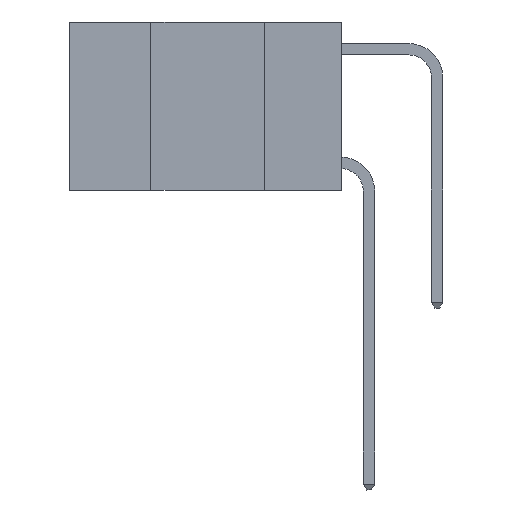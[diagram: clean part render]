
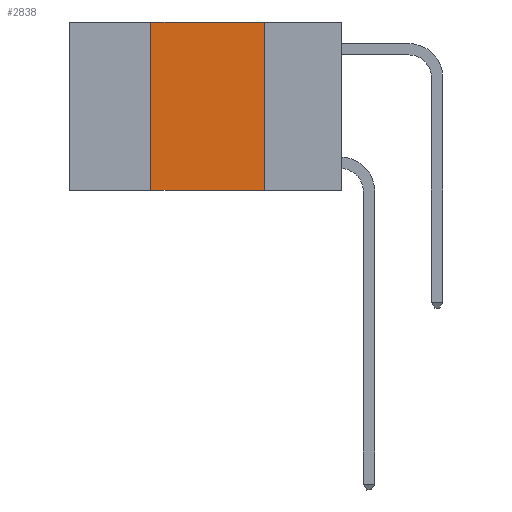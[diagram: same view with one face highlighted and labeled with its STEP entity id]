
A CAD part, left-side view. The second image highlights one B-rep face of the part: STEP entity #2838.
In plain terms, the highlighted planar face has unit normal (-1, 0, 0).
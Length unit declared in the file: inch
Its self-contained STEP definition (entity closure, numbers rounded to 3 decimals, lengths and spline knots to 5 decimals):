
#393 = ORIENTED_EDGE ( 'NONE', *, *, #5896, .T. ) ;
#488 = VECTOR ( 'NONE', #11112, 39.37008 ) ;
#521 = CARTESIAN_POINT ( 'NONE',  ( 0., 0.17, 0. ) ) ;
#688 = ORIENTED_EDGE ( 'NONE', *, *, #948, .F. ) ;
#948 = EDGE_CURVE ( 'NONE', #10338, #5953, #5737, .T. ) ;
#1425 = EDGE_LOOP ( 'NONE', ( #688, #5226, #4576, #393 ) ) ;
#1478 = EDGE_CURVE ( 'NONE', #5827, #5379, #10811, .T. ) ;
#2143 = LINE ( 'NONE', #10212, #6432 ) ;
#2536 = LINE ( 'NONE', #3666, #10911 ) ;
#2667 = DIRECTION ( 'NONE',  ( 0., -1., 0. ) ) ;
#2838 = ADVANCED_FACE ( 'NONE', ( #7087 ), #10651, .F. ) ;
#3084 = CARTESIAN_POINT ( 'NONE',  ( 0., 0.42, 0. ) ) ;
#3153 = CARTESIAN_POINT ( 'NONE',  ( 0., 0.42, 0. ) ) ;
#3666 = CARTESIAN_POINT ( 'NONE',  ( 0., 0.6, -0.37 ) ) ;
#4390 = VECTOR ( 'NONE', #10100, 39.37008 ) ;
#4576 = ORIENTED_EDGE ( 'NONE', *, *, #1478, .F. ) ;
#4587 = EDGE_CURVE ( 'NONE', #5379, #10338, #2143, .T. ) ;
#5131 = CARTESIAN_POINT ( 'NONE',  ( 0., 0.17, -0.37 ) ) ;
#5226 = ORIENTED_EDGE ( 'NONE', *, *, #4587, .F. ) ;
#5379 = VERTEX_POINT ( 'NONE', #3153 ) ;
#5737 = LINE ( 'NONE', #521, #488 ) ;
#5827 = VERTEX_POINT ( 'NONE', #8786 ) ;
#5896 = EDGE_CURVE ( 'NONE', #5827, #5953, #2536, .T. ) ;
#5953 = VERTEX_POINT ( 'NONE', #5131 ) ;
#6352 = CARTESIAN_POINT ( 'NONE',  ( 0., 0.17, 0. ) ) ;
#6432 = VECTOR ( 'NONE', #9313, 39.37008 ) ;
#6895 = CARTESIAN_POINT ( 'NONE',  ( 0., 0.6, 0. ) ) ;
#6956 = DIRECTION ( 'NONE',  ( 0., 0., -1. ) ) ;
#7087 = FACE_OUTER_BOUND ( 'NONE', #1425, .T. ) ;
#8519 = AXIS2_PLACEMENT_3D ( 'NONE', #6895, #10514, #6956 ) ;
#8786 = CARTESIAN_POINT ( 'NONE',  ( 0., 0.42, -0.37 ) ) ;
#9313 = DIRECTION ( 'NONE',  ( 0., -1., 0. ) ) ;
#10100 = DIRECTION ( 'NONE',  ( 0., 0., 1. ) ) ;
#10212 = CARTESIAN_POINT ( 'NONE',  ( 0., 0.6, 0. ) ) ;
#10338 = VERTEX_POINT ( 'NONE', #6352 ) ;
#10514 = DIRECTION ( 'NONE',  ( 1., 0., 0. ) ) ;
#10651 = PLANE ( 'NONE',  #8519 ) ;
#10811 = LINE ( 'NONE', #3084, #4390 ) ;
#10911 = VECTOR ( 'NONE', #2667, 39.37008 ) ;
#11112 = DIRECTION ( 'NONE',  ( 0., 0., -1. ) ) ;
